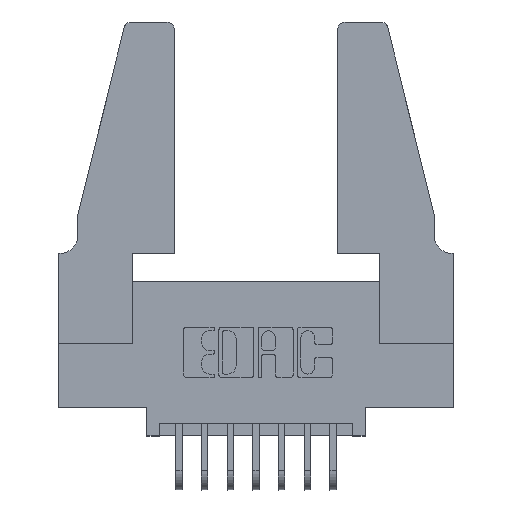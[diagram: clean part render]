
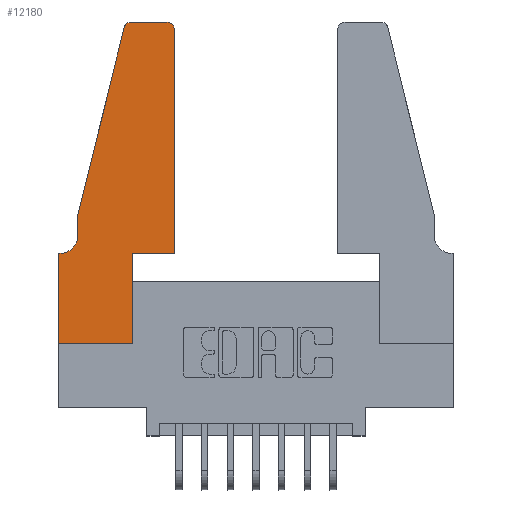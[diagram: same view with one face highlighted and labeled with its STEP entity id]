
A CAD part, top view. The second image highlights one B-rep face of the part: STEP entity #12180.
In plain terms, the highlighted planar face has unit normal (0, 0, 1).
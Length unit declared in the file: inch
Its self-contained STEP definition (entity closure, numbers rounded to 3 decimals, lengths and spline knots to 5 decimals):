
#7 = CARTESIAN_POINT ( 'NONE',  ( 0.0755, 0.5, 0.37 ) ) ;
#429 = CARTESIAN_POINT ( 'NONE',  ( 0., 0.35, 0.37 ) ) ;
#444 = CIRCLE ( 'NONE', #7180, 0.03 ) ;
#476 = DIRECTION ( 'NONE',  ( 1., 0., 0. ) ) ;
#1155 = VERTEX_POINT ( 'NONE', #4162 ) ;
#1360 = CARTESIAN_POINT ( 'NONE',  ( 0.4505, 0.35, 0.37 ) ) ;
#1540 = VECTOR ( 'NONE', #11144, 39.37008 ) ;
#1561 = VECTOR ( 'NONE', #476, 39.37008 ) ;
#1762 = CARTESIAN_POINT ( 'NONE',  ( 0.4505, 0.35, 0.37 ) ) ;
#1828 = LINE ( 'NONE', #2527, #4978 ) ;
#1844 = EDGE_CURVE ( 'NONE', #6695, #5220, #4780, .T. ) ;
#1903 = ORIENTED_EDGE ( 'NONE', *, *, #12332, .T. ) ;
#2119 = CIRCLE ( 'NONE', #6671, 0.03 ) ;
#2332 = PLANE ( 'NONE',  #4516 ) ;
#2350 = VERTEX_POINT ( 'NONE', #5646 ) ;
#2415 = VECTOR ( 'NONE', #3513, 39.37008 ) ;
#2419 = EDGE_CURVE ( 'NONE', #13336, #2350, #6331, .T. ) ;
#2475 = DIRECTION ( 'NONE',  ( -1., 0., 0. ) ) ;
#2482 = VERTEX_POINT ( 'NONE', #11339 ) ;
#2496 = DIRECTION ( 'NONE',  ( 0., 1., 0. ) ) ;
#2527 = CARTESIAN_POINT ( 'NONE',  ( 0.2605, 1.25, 0.37 ) ) ;
#2583 = DIRECTION ( 'NONE',  ( 0., 1., 0. ) ) ;
#2785 = DIRECTION ( 'NONE',  ( -1., 0., 0. ) ) ;
#3100 = CARTESIAN_POINT ( 'NONE',  ( 0.0755, 0.35, 0.37 ) ) ;
#3221 = ORIENTED_EDGE ( 'NONE', *, *, #7919, .T. ) ;
#3313 = VECTOR ( 'NONE', #2496, 39.37008 ) ;
#3355 = CARTESIAN_POINT ( 'NONE',  ( 0.2865, 0.35, 0.37 ) ) ;
#3364 = DIRECTION ( 'NONE',  ( 0., 0., -1. ) ) ;
#3403 = DIRECTION ( 'NONE',  ( -0.239, -0.971, 0. ) ) ;
#3469 = LINE ( 'NONE', #1360, #8942 ) ;
#3513 = DIRECTION ( 'NONE',  ( 1., 0., 0. ) ) ;
#3554 = DIRECTION ( 'NONE',  ( 0., 0., 1. ) ) ;
#3604 = ORIENTED_EDGE ( 'NONE', *, *, #12909, .T. ) ;
#4102 = CARTESIAN_POINT ( 'NONE',  ( 0.4505, 0.35, 0.37 ) ) ;
#4162 = CARTESIAN_POINT ( 'NONE',  ( 0.4205, 1.25, 0.37 ) ) ;
#4298 = CIRCLE ( 'NONE', #11465, 0.07 ) ;
#4323 = ORIENTED_EDGE ( 'NONE', *, *, #9845, .T. ) ;
#4516 = AXIS2_PLACEMENT_3D ( 'NONE', #13071, #3554, #11026 ) ;
#4681 = ORIENTED_EDGE ( 'NONE', *, *, #2419, .T. ) ;
#4780 = LINE ( 'NONE', #3100, #10073 ) ;
#4978 = VECTOR ( 'NONE', #2475, 39.37008 ) ;
#5047 = ORIENTED_EDGE ( 'NONE', *, *, #13076, .T. ) ;
#5220 = VERTEX_POINT ( 'NONE', #429 ) ;
#5377 = DIRECTION ( 'NONE',  ( 0., 0., 1. ) ) ;
#5491 = CARTESIAN_POINT ( 'NONE',  ( 0.0755, 0.5, 0.37 ) ) ;
#5637 = VECTOR ( 'NONE', #7316, 39.37008 ) ;
#5646 = CARTESIAN_POINT ( 'NONE',  ( 0.2865, 0.35, 0.37 ) ) ;
#5753 = CARTESIAN_POINT ( 'NONE',  ( 0.25487, 1.22718, 0.37 ) ) ;
#5841 = CARTESIAN_POINT ( 'NONE',  ( 0.284, 1.22, 0.37 ) ) ;
#5953 = FACE_OUTER_BOUND ( 'NONE', #7563, .T. ) ;
#5998 = CARTESIAN_POINT ( 'NONE',  ( 0.2865, 0., 0.37 ) ) ;
#6029 = VERTEX_POINT ( 'NONE', #5491 ) ;
#6247 = ORIENTED_EDGE ( 'NONE', *, *, #10191, .T. ) ;
#6331 = LINE ( 'NONE', #3355, #3313 ) ;
#6592 = ORIENTED_EDGE ( 'NONE', *, *, #6659, .T. ) ;
#6659 = EDGE_CURVE ( 'NONE', #12429, #6695, #4298, .T. ) ;
#6671 = AXIS2_PLACEMENT_3D ( 'NONE', #11636, #5377, #12689 ) ;
#6695 = VERTEX_POINT ( 'NONE', #8924 ) ;
#6722 = VERTEX_POINT ( 'NONE', #5753 ) ;
#6749 = CARTESIAN_POINT ( 'NONE',  ( 0.0755, 0.5, 0.37 ) ) ;
#6934 = ORIENTED_EDGE ( 'NONE', *, *, #1844, .T. ) ;
#6942 = DIRECTION ( 'NONE',  ( 1., 0., 0. ) ) ;
#7073 = VERTEX_POINT ( 'NONE', #1762 ) ;
#7180 = AXIS2_PLACEMENT_3D ( 'NONE', #5841, #13117, #6942 ) ;
#7247 = CARTESIAN_POINT ( 'NONE',  ( 0.0755, 0.42, 0.37 ) ) ;
#7251 = EDGE_CURVE ( 'NONE', #11095, #13336, #8369, .T. ) ;
#7257 = ORIENTED_EDGE ( 'NONE', *, *, #7251, .T. ) ;
#7316 = DIRECTION ( 'NONE',  ( 0., -1., 0. ) ) ;
#7563 = EDGE_LOOP ( 'NONE', ( #3221, #6247, #11776, #3604, #6592, #6934, #4323, #7257, #4681, #7581, #1903, #5047 ) ) ;
#7581 = ORIENTED_EDGE ( 'NONE', *, *, #10557, .T. ) ;
#7610 = LINE ( 'NONE', #7, #1540 ) ;
#7919 = EDGE_CURVE ( 'NONE', #1155, #2482, #1828, .T. ) ;
#7961 = LINE ( 'NONE', #4102, #1561 ) ;
#8369 = LINE ( 'NONE', #9958, #2415 ) ;
#8654 = VECTOR ( 'NONE', #3403, 39.37008 ) ;
#8924 = CARTESIAN_POINT ( 'NONE',  ( 0.0055, 0.35, 0.37 ) ) ;
#8942 = VECTOR ( 'NONE', #2583, 39.37008 ) ;
#8977 = LINE ( 'NONE', #6749, #8654 ) ;
#8984 = EDGE_CURVE ( 'NONE', #6722, #6029, #8977, .T. ) ;
#9839 = CARTESIAN_POINT ( 'NONE',  ( 0.0055, 0.42, 0.37 ) ) ;
#9845 = EDGE_CURVE ( 'NONE', #5220, #11095, #13918, .T. ) ;
#9958 = CARTESIAN_POINT ( 'NONE',  ( 0., 0., 0.37 ) ) ;
#10073 = VECTOR ( 'NONE', #2785, 39.37008 ) ;
#10191 = EDGE_CURVE ( 'NONE', #2482, #6722, #444, .T. ) ;
#10338 = CARTESIAN_POINT ( 'NONE',  ( 0.4505, 1.22, 0.37 ) ) ;
#10557 = EDGE_CURVE ( 'NONE', #2350, #7073, #7961, .T. ) ;
#10872 = DIRECTION ( 'NONE',  ( -1., 0., 0. ) ) ;
#11026 = DIRECTION ( 'NONE',  ( 1., 0., 0. ) ) ;
#11095 = VERTEX_POINT ( 'NONE', #11470 ) ;
#11144 = DIRECTION ( 'NONE',  ( 0., -1., 0. ) ) ;
#11339 = CARTESIAN_POINT ( 'NONE',  ( 0.284, 1.25, 0.37 ) ) ;
#11408 = CARTESIAN_POINT ( 'NONE',  ( 0., 0., 0.37 ) ) ;
#11465 = AXIS2_PLACEMENT_3D ( 'NONE', #9839, #3364, #10872 ) ;
#11470 = CARTESIAN_POINT ( 'NONE',  ( 0., 0., 0.37 ) ) ;
#11636 = CARTESIAN_POINT ( 'NONE',  ( 0.4205, 1.22, 0.37 ) ) ;
#11776 = ORIENTED_EDGE ( 'NONE', *, *, #8984, .T. ) ;
#12180 = ADVANCED_FACE ( 'NONE', ( #5953 ), #2332, .T. ) ;
#12332 = EDGE_CURVE ( 'NONE', #7073, #14081, #3469, .T. ) ;
#12429 = VERTEX_POINT ( 'NONE', #7247 ) ;
#12689 = DIRECTION ( 'NONE',  ( 1., 0., 0. ) ) ;
#12909 = EDGE_CURVE ( 'NONE', #6029, #12429, #7610, .T. ) ;
#13071 = CARTESIAN_POINT ( 'NONE',  ( 0., 0.35, 0.37 ) ) ;
#13076 = EDGE_CURVE ( 'NONE', #14081, #1155, #2119, .T. ) ;
#13117 = DIRECTION ( 'NONE',  ( 0., 0., 1. ) ) ;
#13336 = VERTEX_POINT ( 'NONE', #5998 ) ;
#13918 = LINE ( 'NONE', #11408, #5637 ) ;
#14081 = VERTEX_POINT ( 'NONE', #10338 ) ;
